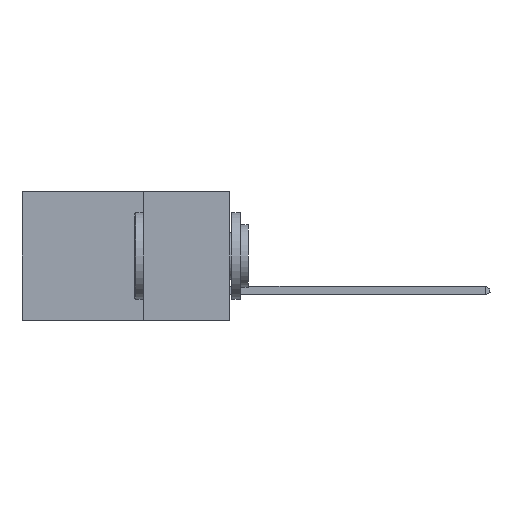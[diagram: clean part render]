
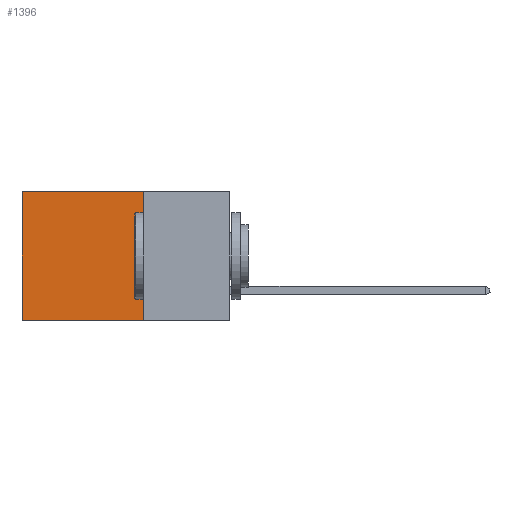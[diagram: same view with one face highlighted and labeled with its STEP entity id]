
A CAD part, left-side view. The second image highlights one B-rep face of the part: STEP entity #1396.
In plain terms, the highlighted planar face has unit normal (-1, 0, 0).
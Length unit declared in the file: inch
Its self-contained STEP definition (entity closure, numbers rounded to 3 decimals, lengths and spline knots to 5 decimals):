
#661 = CARTESIAN_POINT ( 'NONE',  ( 0.298, 0.6, 0. ) ) ;
#995 = CARTESIAN_POINT ( 'NONE',  ( 0.298, 0.25, 0. ) ) ;
#1018 = PLANE ( 'NONE',  #5733 ) ;
#1093 = VECTOR ( 'NONE', #10789, 39.37008 ) ;
#1396 = ADVANCED_FACE ( 'NONE', ( #10035 ), #1018, .F. ) ;
#1510 = LINE ( 'NONE', #2833, #13677 ) ;
#2301 = VERTEX_POINT ( 'NONE', #995 ) ;
#2833 = CARTESIAN_POINT ( 'NONE',  ( 0.298, 0.25, 0. ) ) ;
#2868 = CARTESIAN_POINT ( 'NONE',  ( 0.298, 0.6, -0.37 ) ) ;
#4311 = CARTESIAN_POINT ( 'NONE',  ( 0.298, 0.25, 0. ) ) ;
#4355 = VECTOR ( 'NONE', #4960, 39.37008 ) ;
#4508 = DIRECTION ( 'NONE',  ( 0., 0., -1. ) ) ;
#4960 = DIRECTION ( 'NONE',  ( 0., 0., -1. ) ) ;
#5357 = LINE ( 'NONE', #15589, #1093 ) ;
#5733 = AXIS2_PLACEMENT_3D ( 'NONE', #4311, #6110, #4508 ) ;
#6110 = DIRECTION ( 'NONE',  ( 1., 0., 0. ) ) ;
#7157 = DIRECTION ( 'NONE',  ( 0., 1., 0. ) ) ;
#7406 = VERTEX_POINT ( 'NONE', #661 ) ;
#9264 = VERTEX_POINT ( 'NONE', #13102 ) ;
#9488 = EDGE_CURVE ( 'NONE', #2301, #7406, #1510, .T. ) ;
#10035 = FACE_OUTER_BOUND ( 'NONE', #13982, .T. ) ;
#10789 = DIRECTION ( 'NONE',  ( 0., 1., 0. ) ) ;
#10896 = EDGE_CURVE ( 'NONE', #7406, #19170, #15381, .T. ) ;
#11144 = VECTOR ( 'NONE', #16477, 39.37008 ) ;
#11527 = CARTESIAN_POINT ( 'NONE',  ( 0.298, 0.6, 0. ) ) ;
#12572 = EDGE_CURVE ( 'NONE', #2301, #9264, #20292, .T. ) ;
#13102 = CARTESIAN_POINT ( 'NONE',  ( 0.298, 0.25, -0.37 ) ) ;
#13677 = VECTOR ( 'NONE', #7157, 39.37008 ) ;
#13982 = EDGE_LOOP ( 'NONE', ( #16127, #14330, #16080, #18046 ) ) ;
#14330 = ORIENTED_EDGE ( 'NONE', *, *, #19743, .F. ) ;
#14471 = CARTESIAN_POINT ( 'NONE',  ( 0.298, 0.25, 0. ) ) ;
#15381 = LINE ( 'NONE', #11527, #11144 ) ;
#15589 = CARTESIAN_POINT ( 'NONE',  ( 0.298, 0.25, -0.37 ) ) ;
#16080 = ORIENTED_EDGE ( 'NONE', *, *, #12572, .F. ) ;
#16127 = ORIENTED_EDGE ( 'NONE', *, *, #10896, .T. ) ;
#16477 = DIRECTION ( 'NONE',  ( 0., 0., -1. ) ) ;
#18046 = ORIENTED_EDGE ( 'NONE', *, *, #9488, .T. ) ;
#19170 = VERTEX_POINT ( 'NONE', #2868 ) ;
#19743 = EDGE_CURVE ( 'NONE', #9264, #19170, #5357, .T. ) ;
#20292 = LINE ( 'NONE', #14471, #4355 ) ;
